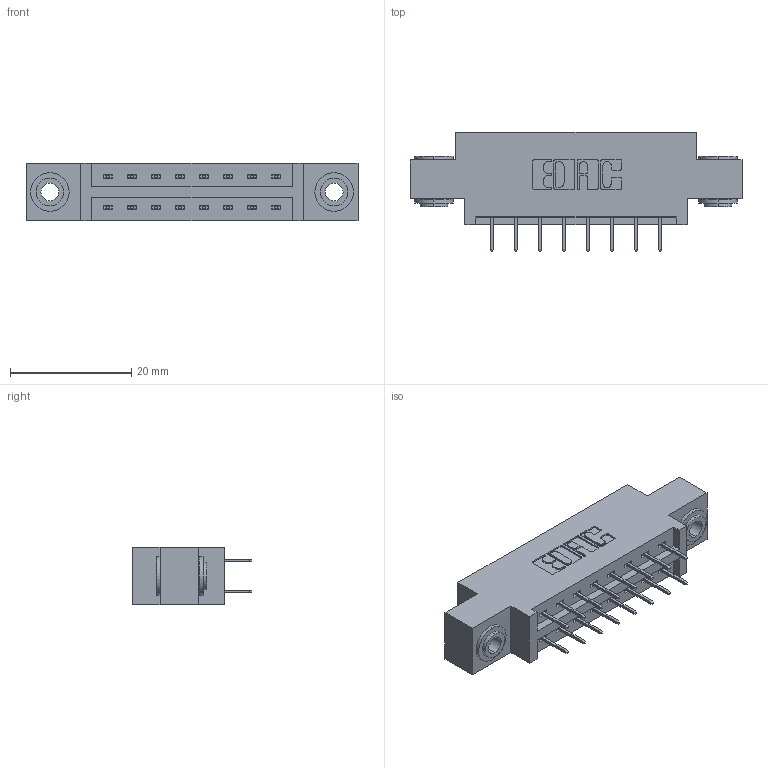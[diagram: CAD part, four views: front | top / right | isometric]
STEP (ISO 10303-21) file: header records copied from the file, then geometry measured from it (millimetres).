
FILE_DESCRIPTION (( 'STEP AP203' ), '1' );
FILE_NAME ('387-016-524-803.STEP', '2019-10-15T22:57:18', ( '' ), ( '' ), 'SwSTEP 2.0', 'SolidWorks 2016', '' );
FILE_SCHEMA (( 'CONFIG_CONTROL_DESIGN' ));
Length unit declared in the file: inch
Products named in the file (4): 337 Part_0.170 Offset - 0.156 Dia-TH; 345-292-001_345-293-124; 387-016-524-803; 345-250-002_345-250-002-102
Assembly tree (19 placements, depth 2):
  387-016-524-803
    337 Part_0.170 Offset - 0.156 Dia-TH
    345-292-001_345-293-124  x16
    345-250-002_345-250-002-102  x2
Bounding box: 54.71 x 19.69 x 9.4 mm (x, y, z)
Volume: 5191 mm3; surface area: 5795.5 mm2
Topology: 19 solids, 19 shells, 1084 faces, 3039 edges, 1958 vertices
Faces by surface type: plane 788, cylinder 288, cone 8
Entity records: 11456 total; most frequent: CARTESIAN_POINT 1933, ORIENTED_EDGE 1862, DIRECTION 1741, EDGE_CURVE 931, VECTOR 783, LINE 783, VERTEX_POINT 614, AXIS2_PLACEMENT_3D 479
